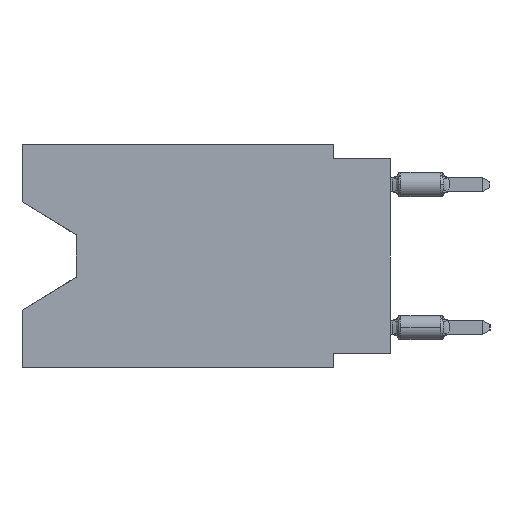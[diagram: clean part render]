
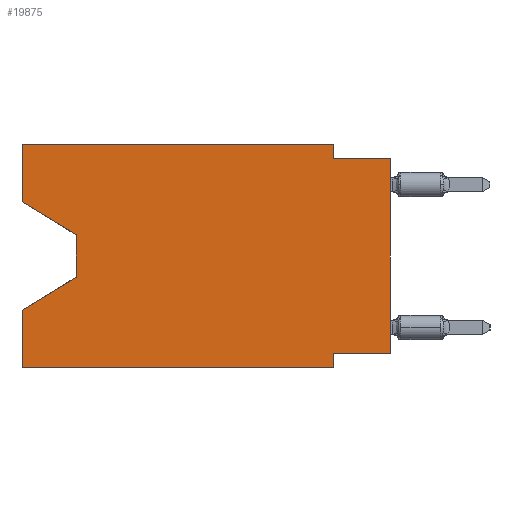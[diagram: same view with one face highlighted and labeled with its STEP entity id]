
A CAD part, left-side view. The second image highlights one B-rep face of the part: STEP entity #19875.
In plain terms, the highlighted planar face has unit normal (-1, 0, 0).
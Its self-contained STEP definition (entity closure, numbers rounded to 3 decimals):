
#107 = ORIENTED_EDGE ( 'NONE', *, *, #4583, .T. ) ;
#984 = VECTOR ( 'NONE', #14876, 1000. ) ;
#1120 = VECTOR ( 'NONE', #33659, 1000. ) ;
#1180 = DIRECTION ( 'NONE',  ( 0., 0.855, -0.519 ) ) ;
#1772 = DIRECTION ( 'NONE',  ( 0., -1., 0. ) ) ;
#2628 = VECTOR ( 'NONE', #18418, 1000. ) ;
#2669 = EDGE_CURVE ( 'NONE', #20910, #7788, #5911, .T. ) ;
#2785 = CARTESIAN_POINT ( 'NONE',  ( 0., 2.54, -9.906 ) ) ;
#3027 = FACE_OUTER_BOUND ( 'NONE', #35176, .T. ) ;
#3223 = CARTESIAN_POINT ( 'NONE',  ( 0., 0., -0.635 ) ) ;
#3288 = CARTESIAN_POINT ( 'NONE',  ( 0., 16.383, -9.906 ) ) ;
#3470 = CARTESIAN_POINT ( 'NONE',  ( 0., 13.97, -4.013 ) ) ;
#3781 = CARTESIAN_POINT ( 'NONE',  ( 0., 0., -0.635 ) ) ;
#3804 = ORIENTED_EDGE ( 'NONE', *, *, #14802, .F. ) ;
#4032 = CARTESIAN_POINT ( 'NONE',  ( 0., 0., -9.271 ) ) ;
#4194 = VERTEX_POINT ( 'NONE', #3470 ) ;
#4583 = EDGE_CURVE ( 'NONE', #35097, #4194, #36212, .T. ) ;
#5034 = ORIENTED_EDGE ( 'NONE', *, *, #18857, .F. ) ;
#5911 = LINE ( 'NONE', #3288, #1120 ) ;
#6778 = LINE ( 'NONE', #18120, #36477 ) ;
#7788 = VERTEX_POINT ( 'NONE', #2785 ) ;
#9709 = CARTESIAN_POINT ( 'NONE',  ( 0., 16.383, 0. ) ) ;
#9743 = DIRECTION ( 'NONE',  ( 0., -1., 0. ) ) ;
#9905 = EDGE_CURVE ( 'NONE', #24260, #19725, #35492, .T. ) ;
#10048 = DIRECTION ( 'NONE',  ( 0., 0., -1. ) ) ;
#10349 = VECTOR ( 'NONE', #28050, 1000. ) ;
#10700 = CARTESIAN_POINT ( 'NONE',  ( 0., 16.383, -2.546 ) ) ;
#12265 = AXIS2_PLACEMENT_3D ( 'NONE', #19969, #28377, #16997 ) ;
#12489 = ORIENTED_EDGE ( 'NONE', *, *, #9905, .F. ) ;
#12599 = CARTESIAN_POINT ( 'NONE',  ( 0., 0., -9.271 ) ) ;
#12892 = DIRECTION ( 'NONE',  ( 0., 0., 1. ) ) ;
#14268 = CARTESIAN_POINT ( 'NONE',  ( 0., 13.97, -5.893 ) ) ;
#14802 = EDGE_CURVE ( 'NONE', #15328, #35219, #24075, .T. ) ;
#14876 = DIRECTION ( 'NONE',  ( 0., 0., 1. ) ) ;
#15328 = VERTEX_POINT ( 'NONE', #16320 ) ;
#15412 = EDGE_CURVE ( 'NONE', #18389, #7788, #23823, .T. ) ;
#16249 = CARTESIAN_POINT ( 'NONE',  ( 0., 16.383, 0. ) ) ;
#16320 = CARTESIAN_POINT ( 'NONE',  ( 0., 2.54, -0.635 ) ) ;
#16997 = DIRECTION ( 'NONE',  ( 0., 0., -1. ) ) ;
#17455 = CARTESIAN_POINT ( 'NONE',  ( 0., 16.383, -9.906 ) ) ;
#17853 = EDGE_CURVE ( 'NONE', #22148, #18389, #34635, .T. ) ;
#18039 = LINE ( 'NONE', #26617, #23418 ) ;
#18114 = EDGE_CURVE ( 'NONE', #4194, #34406, #33830, .T. ) ;
#18120 = CARTESIAN_POINT ( 'NONE',  ( 0., 13.97, -5.893 ) ) ;
#18389 = VERTEX_POINT ( 'NONE', #27266 ) ;
#18418 = DIRECTION ( 'NONE',  ( 0., 0., -1. ) ) ;
#18543 = EDGE_CURVE ( 'NONE', #20910, #30004, #19223, .T. ) ;
#18857 = EDGE_CURVE ( 'NONE', #35097, #24260, #26845, .T. ) ;
#19205 = ORIENTED_EDGE ( 'NONE', *, *, #18543, .F. ) ;
#19223 = LINE ( 'NONE', #16249, #19285 ) ;
#19285 = VECTOR ( 'NONE', #30986, 1000. ) ;
#19526 = CARTESIAN_POINT ( 'NONE',  ( 0., 16.383, -7.36 ) ) ;
#19725 = VERTEX_POINT ( 'NONE', #33382 ) ;
#19754 = ORIENTED_EDGE ( 'NONE', *, *, #17853, .F. ) ;
#19875 = ADVANCED_FACE ( 'NONE', ( #3027 ), #36740, .F. ) ;
#19969 = CARTESIAN_POINT ( 'NONE',  ( 0., 16.383, 0. ) ) ;
#20175 = VECTOR ( 'NONE', #22034, 1000. ) ;
#20475 = EDGE_CURVE ( 'NONE', #22148, #35219, #21000, .T. ) ;
#20910 = VERTEX_POINT ( 'NONE', #17455 ) ;
#21000 = LINE ( 'NONE', #23261, #984 ) ;
#21011 = VECTOR ( 'NONE', #9743, 1000. ) ;
#22034 = DIRECTION ( 'NONE',  ( 0., -0.855, -0.519 ) ) ;
#22148 = VERTEX_POINT ( 'NONE', #4032 ) ;
#22754 = ORIENTED_EDGE ( 'NONE', *, *, #15412, .F. ) ;
#22897 = VECTOR ( 'NONE', #12892, 1000. ) ;
#23261 = CARTESIAN_POINT ( 'NONE',  ( 0., 0., 0. ) ) ;
#23418 = VECTOR ( 'NONE', #10048, 1000. ) ;
#23785 = EDGE_CURVE ( 'NONE', #34406, #30004, #6778, .T. ) ;
#23823 = LINE ( 'NONE', #29431, #2628 ) ;
#23861 = CARTESIAN_POINT ( 'NONE',  ( 0., 16.383, 0. ) ) ;
#24075 = LINE ( 'NONE', #3781, #21011 ) ;
#24260 = VERTEX_POINT ( 'NONE', #9709 ) ;
#24614 = VECTOR ( 'NONE', #28882, 1000. ) ;
#26617 = CARTESIAN_POINT ( 'NONE',  ( 0., 2.54, 0. ) ) ;
#26845 = LINE ( 'NONE', #23861, #22897 ) ;
#27072 = ORIENTED_EDGE ( 'NONE', *, *, #23785, .T. ) ;
#27266 = CARTESIAN_POINT ( 'NONE',  ( 0., 2.54, -9.271 ) ) ;
#27287 = CARTESIAN_POINT ( 'NONE',  ( 0., 16.383, 0. ) ) ;
#27823 = VECTOR ( 'NONE', #1772, 1000. ) ;
#28050 = DIRECTION ( 'NONE',  ( 0., 0., -1. ) ) ;
#28377 = DIRECTION ( 'NONE',  ( 1., 0., 0. ) ) ;
#28734 = ORIENTED_EDGE ( 'NONE', *, *, #18114, .T. ) ;
#28882 = DIRECTION ( 'NONE',  ( 0., 1., 0. ) ) ;
#29431 = CARTESIAN_POINT ( 'NONE',  ( 0., 2.54, -9.906 ) ) ;
#30004 = VERTEX_POINT ( 'NONE', #19526 ) ;
#30417 = CARTESIAN_POINT ( 'NONE',  ( 0., 16.383, -2.546 ) ) ;
#30986 = DIRECTION ( 'NONE',  ( 0., 0., 1. ) ) ;
#32252 = ORIENTED_EDGE ( 'NONE', *, *, #20475, .T. ) ;
#32460 = EDGE_CURVE ( 'NONE', #19725, #15328, #18039, .T. ) ;
#33382 = CARTESIAN_POINT ( 'NONE',  ( 0., 2.54, 0. ) ) ;
#33659 = DIRECTION ( 'NONE',  ( 0., -1., 0. ) ) ;
#33830 = LINE ( 'NONE', #36227, #10349 ) ;
#34406 = VERTEX_POINT ( 'NONE', #14268 ) ;
#34635 = LINE ( 'NONE', #12599, #24614 ) ;
#34806 = ORIENTED_EDGE ( 'NONE', *, *, #2669, .T. ) ;
#34832 = ORIENTED_EDGE ( 'NONE', *, *, #32460, .F. ) ;
#35097 = VERTEX_POINT ( 'NONE', #30417 ) ;
#35176 = EDGE_LOOP ( 'NONE', ( #107, #28734, #27072, #19205, #34806, #22754, #19754, #32252, #3804, #34832, #12489, #5034 ) ) ;
#35219 = VERTEX_POINT ( 'NONE', #3223 ) ;
#35492 = LINE ( 'NONE', #27287, #27823 ) ;
#36212 = LINE ( 'NONE', #10700, #20175 ) ;
#36227 = CARTESIAN_POINT ( 'NONE',  ( 0., 13.97, -4.013 ) ) ;
#36477 = VECTOR ( 'NONE', #1180, 1000. ) ;
#36740 = PLANE ( 'NONE',  #12265 ) ;
